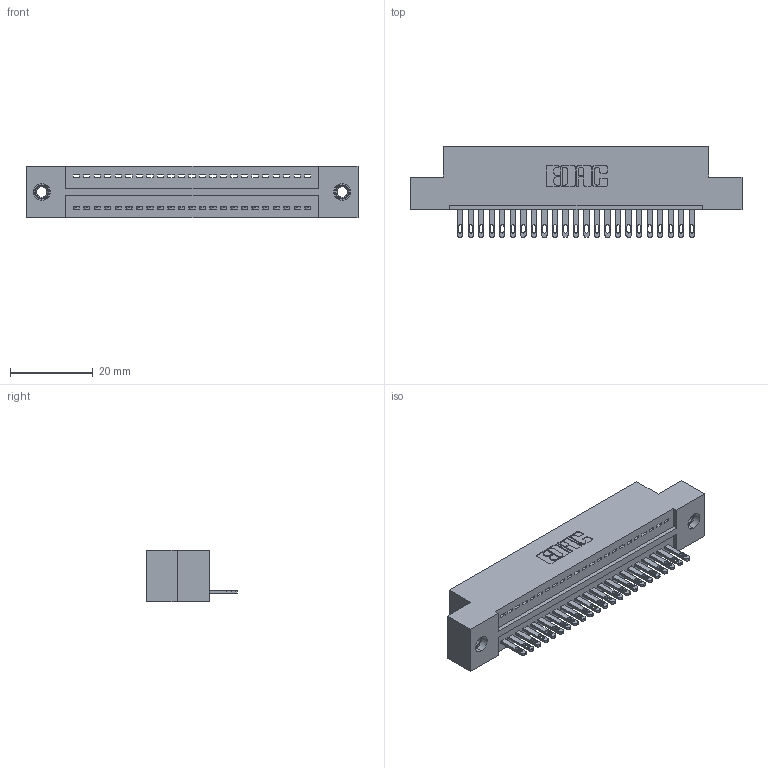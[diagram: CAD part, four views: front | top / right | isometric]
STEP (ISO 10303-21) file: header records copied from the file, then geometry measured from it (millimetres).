
FILE_DESCRIPTION (( 'STEP AP203' ), '1' );
FILE_NAME ('325-023-500-107.STEP', '2020-02-24T17:36:05', ( '' ), ( '' ), 'SwSTEP 2.0', 'SolidWorks 2016', '' );
FILE_SCHEMA (( 'CONFIG_CONTROL_DESIGN' ));
Length unit declared in the file: inch
Products named in the file (4): 345-250-001_345-250-005-103; 325 Part_TI; 325-023-500-107; 325-292-001_325-293-100
Assembly tree (26 placements, depth 2):
  325-023-500-107
    325 Part_TI
    325-292-001_325-293-100  x23
    345-250-001_345-250-005-103  x2
Bounding box: 80.14 x 21.84 x 12.45 mm (x, y, z)
Volume: 10024.7 mm3; surface area: 10710.7 mm2
Topology: 26 solids, 26 shells, 1416 faces, 4311 edges, 2866 vertices
Faces by surface type: plane 930, cylinder 470, cone 12, torus 4
Entity records: 17634 total; most frequent: CARTESIAN_POINT 3026, ORIENTED_EDGE 2978, DIRECTION 2625, EDGE_CURVE 1489, LINE 1337, VECTOR 1337, VERTEX_POINT 988, AXIS2_PLACEMENT_3D 644
